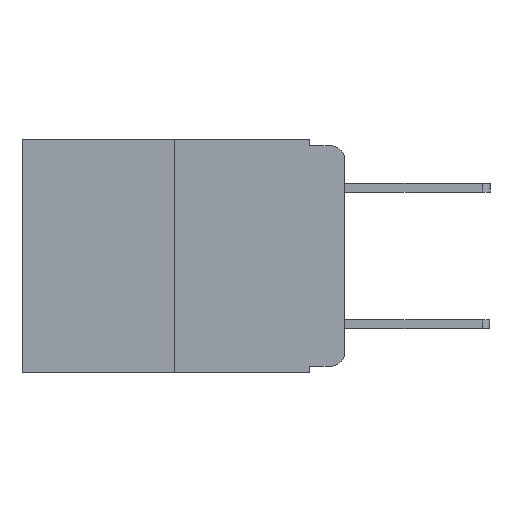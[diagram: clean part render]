
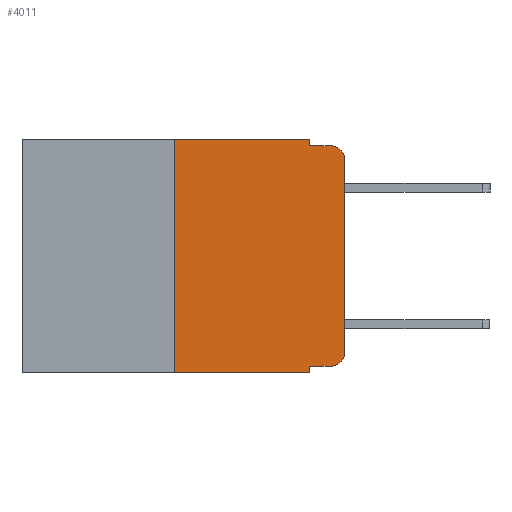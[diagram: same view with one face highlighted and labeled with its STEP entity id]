
A CAD part, left-side view. The second image highlights one B-rep face of the part: STEP entity #4011.
In plain terms, the highlighted planar face has unit normal (-1, 0, 0).
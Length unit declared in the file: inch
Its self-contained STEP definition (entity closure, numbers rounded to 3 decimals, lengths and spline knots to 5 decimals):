
#3 = VECTOR ( 'NONE', #15004, 39.37008 ) ;
#131 = VECTOR ( 'NONE', #22800, 39.37008 ) ;
#482 = VERTEX_POINT ( 'NONE', #15907 ) ;
#610 = VECTOR ( 'NONE', #13276, 39.37008 ) ;
#900 = LINE ( 'NONE', #17924, #11054 ) ;
#1020 = DIRECTION ( 'NONE',  ( -1., 0., 0. ) ) ;
#1297 = VECTOR ( 'NONE', #22907, 39.37008 ) ;
#1482 = EDGE_CURVE ( 'NONE', #16622, #17374, #21243, .T. ) ;
#1840 = VERTEX_POINT ( 'NONE', #23860 ) ;
#2061 = ORIENTED_EDGE ( 'NONE', *, *, #12982, .F. ) ;
#2076 = FACE_OUTER_BOUND ( 'NONE', #12904, .T. ) ;
#2220 = VERTEX_POINT ( 'NONE', #13852 ) ;
#2555 = VERTEX_POINT ( 'NONE', #16495 ) ;
#2993 = DIRECTION ( 'NONE',  ( 0., 0., 1. ) ) ;
#3390 = CARTESIAN_POINT ( 'NONE',  ( 0., 0.25, 0. ) ) ;
#3573 = EDGE_CURVE ( 'NONE', #6386, #21025, #900, .T. ) ;
#3838 = AXIS2_PLACEMENT_3D ( 'NONE', #6561, #17804, #6649 ) ;
#4011 = ADVANCED_FACE ( 'NONE', ( #2076 ), #21418, .F. ) ;
#4976 = EDGE_CURVE ( 'NONE', #17626, #2555, #19477, .T. ) ;
#5070 = ORIENTED_EDGE ( 'NONE', *, *, #4976, .F. ) ;
#5308 = LINE ( 'NONE', #17247, #131 ) ;
#5311 = DIRECTION ( 'NONE',  ( 0., 0., 1. ) ) ;
#5590 = VECTOR ( 'NONE', #17096, 39.37008 ) ;
#5668 = ORIENTED_EDGE ( 'NONE', *, *, #11246, .T. ) ;
#5676 = ORIENTED_EDGE ( 'NONE', *, *, #1482, .F. ) ;
#5757 = CARTESIAN_POINT ( 'NONE',  ( 0., 0.051, -0.01 ) ) ;
#5925 = CARTESIAN_POINT ( 'NONE',  ( 0., 0.051, 0. ) ) ;
#5933 = ORIENTED_EDGE ( 'NONE', *, *, #17945, .T. ) ;
#6251 = LINE ( 'NONE', #3390, #11281 ) ;
#6297 = ORIENTED_EDGE ( 'NONE', *, *, #21397, .F. ) ;
#6386 = VERTEX_POINT ( 'NONE', #8288 ) ;
#6561 = CARTESIAN_POINT ( 'NONE',  ( 0., 0.473, 0. ) ) ;
#6649 = DIRECTION ( 'NONE',  ( 0., 0., -1. ) ) ;
#6812 = DIRECTION ( 'NONE',  ( -1., 0., 0. ) ) ;
#8288 = CARTESIAN_POINT ( 'NONE',  ( 0., 0.051, -0.333 ) ) ;
#8591 = DIRECTION ( 'NONE',  ( 0., -1., 0. ) ) ;
#9424 = LINE ( 'NONE', #5925, #5590 ) ;
#10788 = LINE ( 'NONE', #11427, #610 ) ;
#11054 = VECTOR ( 'NONE', #8591, 39.37008 ) ;
#11246 = EDGE_CURVE ( 'NONE', #21025, #19398, #14535, .T. ) ;
#11281 = VECTOR ( 'NONE', #5311, 39.37008 ) ;
#11427 = CARTESIAN_POINT ( 'NONE',  ( 0., 0.051, 0. ) ) ;
#12411 = CARTESIAN_POINT ( 'NONE',  ( 0., 0.02, -0.03 ) ) ;
#12904 = EDGE_LOOP ( 'NONE', ( #17897, #5933, #5070, #19075, #5676, #2061, #19965, #6297, #19374, #5668 ) ) ;
#12982 = EDGE_CURVE ( 'NONE', #1840, #16622, #6251, .T. ) ;
#13150 = CARTESIAN_POINT ( 'NONE',  ( 0., 0.051, -0.01 ) ) ;
#13276 = DIRECTION ( 'NONE',  ( 0., 0., -1. ) ) ;
#13443 = LINE ( 'NONE', #16121, #14025 ) ;
#13731 = CARTESIAN_POINT ( 'NONE',  ( 0., 0.473, 0. ) ) ;
#13852 = CARTESIAN_POINT ( 'NONE',  ( 0., 0.051, -0.343 ) ) ;
#14025 = VECTOR ( 'NONE', #2993, 39.37008 ) ;
#14131 = EDGE_CURVE ( 'NONE', #1840, #2220, #5308, .T. ) ;
#14258 = DIRECTION ( 'NONE',  ( 0., 0., -1. ) ) ;
#14535 = CIRCLE ( 'NONE', #22651, 0.02 ) ;
#15004 = DIRECTION ( 'NONE',  ( 0., -1., 0. ) ) ;
#15907 = CARTESIAN_POINT ( 'NONE',  ( 0., 0., -0.03 ) ) ;
#16070 = CARTESIAN_POINT ( 'NONE',  ( 0., 0.02, -0.333 ) ) ;
#16121 = CARTESIAN_POINT ( 'NONE',  ( 0., 0., 0. ) ) ;
#16215 = CARTESIAN_POINT ( 'NONE',  ( 0., 0.051, 0. ) ) ;
#16495 = CARTESIAN_POINT ( 'NONE',  ( 0., 0.02, -0.01 ) ) ;
#16622 = VERTEX_POINT ( 'NONE', #22160 ) ;
#17096 = DIRECTION ( 'NONE',  ( 0., 0., -1. ) ) ;
#17247 = CARTESIAN_POINT ( 'NONE',  ( 0., 0.473, -0.343 ) ) ;
#17374 = VERTEX_POINT ( 'NONE', #16215 ) ;
#17626 = VERTEX_POINT ( 'NONE', #5757 ) ;
#17804 = DIRECTION ( 'NONE',  ( 1., 0., 0. ) ) ;
#17897 = ORIENTED_EDGE ( 'NONE', *, *, #23649, .T. ) ;
#17924 = CARTESIAN_POINT ( 'NONE',  ( 0., 0.051, -0.333 ) ) ;
#17945 = EDGE_CURVE ( 'NONE', #482, #2555, #22286, .T. ) ;
#17977 = CARTESIAN_POINT ( 'NONE',  ( 0., 0.02, -0.313 ) ) ;
#18242 = EDGE_CURVE ( 'NONE', #17374, #17626, #10788, .T. ) ;
#18428 = AXIS2_PLACEMENT_3D ( 'NONE', #12411, #1020, #14258 ) ;
#19075 = ORIENTED_EDGE ( 'NONE', *, *, #18242, .F. ) ;
#19374 = ORIENTED_EDGE ( 'NONE', *, *, #3573, .T. ) ;
#19398 = VERTEX_POINT ( 'NONE', #20479 ) ;
#19477 = LINE ( 'NONE', #13150, #3 ) ;
#19828 = DIRECTION ( 'NONE',  ( 0., 0., -1. ) ) ;
#19965 = ORIENTED_EDGE ( 'NONE', *, *, #14131, .T. ) ;
#20479 = CARTESIAN_POINT ( 'NONE',  ( 0., 0., -0.313 ) ) ;
#21025 = VERTEX_POINT ( 'NONE', #16070 ) ;
#21243 = LINE ( 'NONE', #13731, #1297 ) ;
#21397 = EDGE_CURVE ( 'NONE', #6386, #2220, #9424, .T. ) ;
#21418 = PLANE ( 'NONE',  #3838 ) ;
#22160 = CARTESIAN_POINT ( 'NONE',  ( 0., 0.25, 0. ) ) ;
#22286 = CIRCLE ( 'NONE', #18428, 0.02 ) ;
#22651 = AXIS2_PLACEMENT_3D ( 'NONE', #17977, #6812, #19828 ) ;
#22800 = DIRECTION ( 'NONE',  ( 0., -1., 0. ) ) ;
#22907 = DIRECTION ( 'NONE',  ( 0., -1., 0. ) ) ;
#23649 = EDGE_CURVE ( 'NONE', #19398, #482, #13443, .T. ) ;
#23860 = CARTESIAN_POINT ( 'NONE',  ( 0., 0.25, -0.343 ) ) ;
